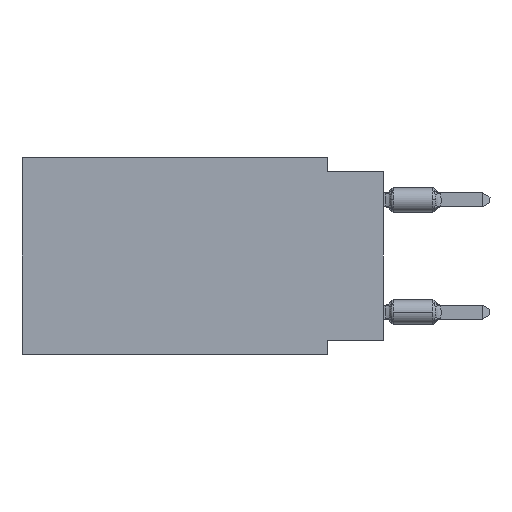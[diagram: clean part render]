
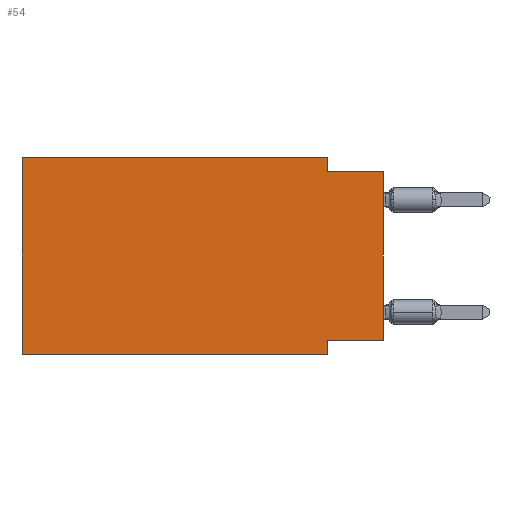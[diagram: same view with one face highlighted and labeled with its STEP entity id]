
A CAD part, left-side view. The second image highlights one B-rep face of the part: STEP entity #54.
In plain terms, the highlighted planar face has unit normal (-1, 0, 0).
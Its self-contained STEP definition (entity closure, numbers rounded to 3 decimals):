
#54 = ADVANCED_FACE ( 'NONE', ( #9699 ), #1298, .F. ) ;
#525 = EDGE_LOOP ( 'NONE', ( #10854, #6838, #12701, #5180, #4282, #12781, #13349, #13058 ) ) ;
#728 = VECTOR ( 'NONE', #4295, 1000. ) ;
#855 = VECTOR ( 'NONE', #12597, 1000. ) ;
#1086 = VERTEX_POINT ( 'NONE', #3648 ) ;
#1170 = EDGE_CURVE ( 'NONE', #1086, #3755, #3088, .T. ) ;
#1298 = PLANE ( 'NONE',  #6052 ) ;
#1551 = CARTESIAN_POINT ( 'NONE',  ( 0., 2.54, 0. ) ) ;
#1604 = CARTESIAN_POINT ( 'NONE',  ( 0., 0., -0.635 ) ) ;
#1616 = DIRECTION ( 'NONE',  ( 0., 0., -1. ) ) ;
#1717 = CARTESIAN_POINT ( 'NONE',  ( 0., 0., -0.635 ) ) ;
#1793 = CARTESIAN_POINT ( 'NONE',  ( 0., 16.383, 0. ) ) ;
#1802 = VERTEX_POINT ( 'NONE', #7977 ) ;
#2095 = VECTOR ( 'NONE', #1616, 1000. ) ;
#2186 = EDGE_CURVE ( 'NONE', #7058, #5275, #2497, .T. ) ;
#2339 = DIRECTION ( 'NONE',  ( 0., 0., -1. ) ) ;
#2497 = LINE ( 'NONE', #1551, #2095 ) ;
#2768 = VECTOR ( 'NONE', #5756, 1000. ) ;
#2813 = LINE ( 'NONE', #1793, #11760 ) ;
#3011 = VECTOR ( 'NONE', #6164, 1000. ) ;
#3088 = LINE ( 'NONE', #10273, #3011 ) ;
#3267 = DIRECTION ( 'NONE',  ( 1., 0., 0. ) ) ;
#3648 = CARTESIAN_POINT ( 'NONE',  ( 0., 0., -8.255 ) ) ;
#3755 = VERTEX_POINT ( 'NONE', #1717 ) ;
#4034 = DIRECTION ( 'NONE',  ( 0., -1., 0. ) ) ;
#4282 = ORIENTED_EDGE ( 'NONE', *, *, #5030, .F. ) ;
#4295 = DIRECTION ( 'NONE',  ( 0., 1., 0. ) ) ;
#4577 = VERTEX_POINT ( 'NONE', #12931 ) ;
#5030 = EDGE_CURVE ( 'NONE', #7523, #4577, #8758, .T. ) ;
#5180 = ORIENTED_EDGE ( 'NONE', *, *, #13249, .F. ) ;
#5275 = VERTEX_POINT ( 'NONE', #9621 ) ;
#5358 = CARTESIAN_POINT ( 'NONE',  ( 0., 16.383, -8.89 ) ) ;
#5382 = DIRECTION ( 'NONE',  ( 0., 0., -1. ) ) ;
#5756 = DIRECTION ( 'NONE',  ( 0., -1., 0. ) ) ;
#6005 = VECTOR ( 'NONE', #2339, 1000. ) ;
#6052 = AXIS2_PLACEMENT_3D ( 'NONE', #8738, #3267, #5382 ) ;
#6055 = EDGE_CURVE ( 'NONE', #1802, #9310, #11551, .T. ) ;
#6164 = DIRECTION ( 'NONE',  ( 0., 0., 1. ) ) ;
#6598 = CARTESIAN_POINT ( 'NONE',  ( 0., 16.383, -8.89 ) ) ;
#6838 = ORIENTED_EDGE ( 'NONE', *, *, #6958, .F. ) ;
#6958 = EDGE_CURVE ( 'NONE', #5275, #3755, #11902, .T. ) ;
#7058 = VERTEX_POINT ( 'NONE', #11336 ) ;
#7523 = VERTEX_POINT ( 'NONE', #5358 ) ;
#7977 = CARTESIAN_POINT ( 'NONE',  ( 0., 2.54, -8.255 ) ) ;
#8063 = DIRECTION ( 'NONE',  ( 0., 0., 1. ) ) ;
#8371 = VECTOR ( 'NONE', #8063, 1000. ) ;
#8437 = LINE ( 'NONE', #6598, #855 ) ;
#8738 = CARTESIAN_POINT ( 'NONE',  ( 0., 16.383, 0. ) ) ;
#8758 = LINE ( 'NONE', #10946, #8371 ) ;
#9310 = VERTEX_POINT ( 'NONE', #10137 ) ;
#9621 = CARTESIAN_POINT ( 'NONE',  ( 0., 2.54, -0.635 ) ) ;
#9625 = CARTESIAN_POINT ( 'NONE',  ( 0., 0., -8.255 ) ) ;
#9699 = FACE_OUTER_BOUND ( 'NONE', #525, .T. ) ;
#9915 = EDGE_CURVE ( 'NONE', #1086, #1802, #13252, .T. ) ;
#10137 = CARTESIAN_POINT ( 'NONE',  ( 0., 2.54, -8.89 ) ) ;
#10273 = CARTESIAN_POINT ( 'NONE',  ( 0., 0., 0. ) ) ;
#10854 = ORIENTED_EDGE ( 'NONE', *, *, #1170, .T. ) ;
#10946 = CARTESIAN_POINT ( 'NONE',  ( 0., 16.383, 0. ) ) ;
#11336 = CARTESIAN_POINT ( 'NONE',  ( 0., 2.54, 0. ) ) ;
#11551 = LINE ( 'NONE', #12716, #6005 ) ;
#11760 = VECTOR ( 'NONE', #4034, 1000. ) ;
#11902 = LINE ( 'NONE', #1604, #2768 ) ;
#12170 = EDGE_CURVE ( 'NONE', #7523, #9310, #8437, .T. ) ;
#12597 = DIRECTION ( 'NONE',  ( 0., -1., 0. ) ) ;
#12701 = ORIENTED_EDGE ( 'NONE', *, *, #2186, .F. ) ;
#12716 = CARTESIAN_POINT ( 'NONE',  ( 0., 2.54, -8.89 ) ) ;
#12781 = ORIENTED_EDGE ( 'NONE', *, *, #12170, .T. ) ;
#12931 = CARTESIAN_POINT ( 'NONE',  ( 0., 16.383, 0. ) ) ;
#13058 = ORIENTED_EDGE ( 'NONE', *, *, #9915, .F. ) ;
#13249 = EDGE_CURVE ( 'NONE', #4577, #7058, #2813, .T. ) ;
#13252 = LINE ( 'NONE', #9625, #728 ) ;
#13349 = ORIENTED_EDGE ( 'NONE', *, *, #6055, .F. ) ;
